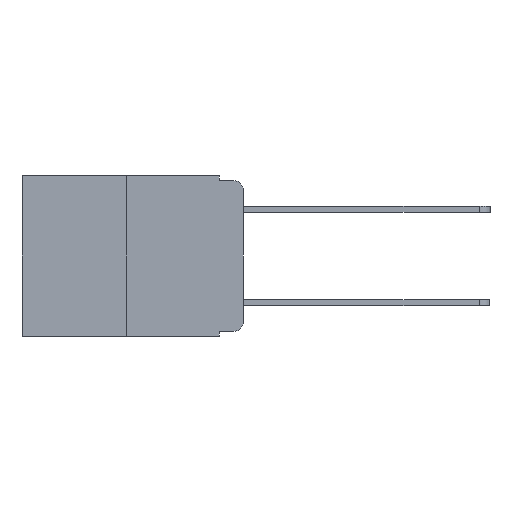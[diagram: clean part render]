
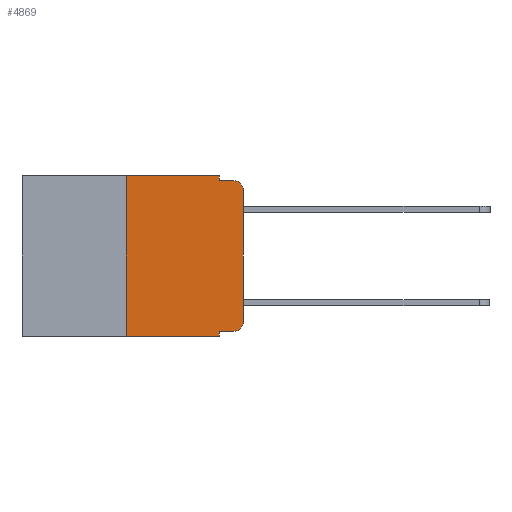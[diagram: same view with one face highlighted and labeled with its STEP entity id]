
A CAD part, left-side view. The second image highlights one B-rep face of the part: STEP entity #4869.
In plain terms, the highlighted planar face has unit normal (-1, 0, 0).
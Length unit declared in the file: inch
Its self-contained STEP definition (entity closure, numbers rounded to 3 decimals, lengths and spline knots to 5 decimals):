
#511 = LINE ( 'NONE', #5958, #3139 ) ;
#607 = ORIENTED_EDGE ( 'NONE', *, *, #5416, .T. ) ;
#632 = CARTESIAN_POINT ( 'NONE',  ( 0., 0.473, -0.343 ) ) ;
#1152 = VERTEX_POINT ( 'NONE', #1390 ) ;
#1154 = DIRECTION ( 'NONE',  ( 0., 0., -1. ) ) ;
#1282 = VERTEX_POINT ( 'NONE', #6256 ) ;
#1390 = CARTESIAN_POINT ( 'NONE',  ( 0., 0.02, -0.333 ) ) ;
#1535 = VECTOR ( 'NONE', #2801, 39.37008 ) ;
#1719 = EDGE_CURVE ( 'NONE', #7092, #6377, #4460, .T. ) ;
#1879 = VERTEX_POINT ( 'NONE', #2275 ) ;
#1970 = VECTOR ( 'NONE', #10909, 39.37008 ) ;
#1979 = CARTESIAN_POINT ( 'NONE',  ( 0., 0.02, -0.03 ) ) ;
#2105 = CARTESIAN_POINT ( 'NONE',  ( 0., 0.051, -0.343 ) ) ;
#2164 = CARTESIAN_POINT ( 'NONE',  ( 0., 0.051, -0.333 ) ) ;
#2275 = CARTESIAN_POINT ( 'NONE',  ( 0., 0.25, 0. ) ) ;
#2300 = AXIS2_PLACEMENT_3D ( 'NONE', #13156, #7542, #1154 ) ;
#2321 = CARTESIAN_POINT ( 'NONE',  ( 0., 0.051, -0.01 ) ) ;
#2801 = DIRECTION ( 'NONE',  ( 0., -1., 0. ) ) ;
#2997 = VERTEX_POINT ( 'NONE', #6821 ) ;
#3131 = VECTOR ( 'NONE', #5124, 39.37008 ) ;
#3139 = VECTOR ( 'NONE', #6002, 39.37008 ) ;
#3471 = CARTESIAN_POINT ( 'NONE',  ( 0., 0., -0.313 ) ) ;
#3485 = VERTEX_POINT ( 'NONE', #12842 ) ;
#3755 = PLANE ( 'NONE',  #7483 ) ;
#3914 = EDGE_CURVE ( 'NONE', #5323, #6377, #9899, .T. ) ;
#4236 = EDGE_LOOP ( 'NONE', ( #607, #6588, #8258, #5287, #4582, #8567, #7348, #9605, #12849, #6663 ) ) ;
#4460 = LINE ( 'NONE', #13046, #1535 ) ;
#4582 = ORIENTED_EDGE ( 'NONE', *, *, #7466, .F. ) ;
#4869 = ADVANCED_FACE ( 'NONE', ( #8647 ), #3755, .F. ) ;
#4973 = CARTESIAN_POINT ( 'NONE',  ( 0., 0., -0.03 ) ) ;
#5023 = VECTOR ( 'NONE', #10057, 39.37008 ) ;
#5072 = VECTOR ( 'NONE', #9431, 39.37008 ) ;
#5124 = DIRECTION ( 'NONE',  ( 0., 0., -1. ) ) ;
#5231 = LINE ( 'NONE', #9103, #1970 ) ;
#5278 = CIRCLE ( 'NONE', #2300, 0.02 ) ;
#5287 = ORIENTED_EDGE ( 'NONE', *, *, #12079, .F. ) ;
#5323 = VERTEX_POINT ( 'NONE', #4973 ) ;
#5416 = EDGE_CURVE ( 'NONE', #8509, #5323, #9421, .T. ) ;
#5656 = CARTESIAN_POINT ( 'NONE',  ( 0., 0., 0. ) ) ;
#5958 = CARTESIAN_POINT ( 'NONE',  ( 0., 0.25, 0. ) ) ;
#6002 = DIRECTION ( 'NONE',  ( 0., 0., 1. ) ) ;
#6009 = LINE ( 'NONE', #8120, #3131 ) ;
#6147 = CARTESIAN_POINT ( 'NONE',  ( 0., 0.473, 0. ) ) ;
#6256 = CARTESIAN_POINT ( 'NONE',  ( 0., 0.051, 0. ) ) ;
#6377 = VERTEX_POINT ( 'NONE', #7809 ) ;
#6547 = DIRECTION ( 'NONE',  ( 1., 0., 0. ) ) ;
#6588 = ORIENTED_EDGE ( 'NONE', *, *, #3914, .T. ) ;
#6663 = ORIENTED_EDGE ( 'NONE', *, *, #7675, .T. ) ;
#6821 = CARTESIAN_POINT ( 'NONE',  ( 0., 0.051, -0.333 ) ) ;
#7092 = VERTEX_POINT ( 'NONE', #2321 ) ;
#7214 = CARTESIAN_POINT ( 'NONE',  ( 0., 0.473, 0. ) ) ;
#7348 = ORIENTED_EDGE ( 'NONE', *, *, #10941, .T. ) ;
#7422 = VECTOR ( 'NONE', #12330, 39.37008 ) ;
#7466 = EDGE_CURVE ( 'NONE', #1879, #1282, #10366, .T. ) ;
#7483 = AXIS2_PLACEMENT_3D ( 'NONE', #6147, #6547, #7631 ) ;
#7542 = DIRECTION ( 'NONE',  ( -1., 0., 0. ) ) ;
#7631 = DIRECTION ( 'NONE',  ( 0., 0., -1. ) ) ;
#7675 = EDGE_CURVE ( 'NONE', #1152, #8509, #5278, .T. ) ;
#7781 = LINE ( 'NONE', #2164, #5072 ) ;
#7809 = CARTESIAN_POINT ( 'NONE',  ( 0., 0.02, -0.01 ) ) ;
#8120 = CARTESIAN_POINT ( 'NONE',  ( 0., 0.051, 0. ) ) ;
#8258 = ORIENTED_EDGE ( 'NONE', *, *, #1719, .F. ) ;
#8334 = EDGE_CURVE ( 'NONE', #2997, #1152, #7781, .T. ) ;
#8509 = VERTEX_POINT ( 'NONE', #3471 ) ;
#8517 = AXIS2_PLACEMENT_3D ( 'NONE', #1979, #10623, #10744 ) ;
#8567 = ORIENTED_EDGE ( 'NONE', *, *, #10856, .F. ) ;
#8647 = FACE_OUTER_BOUND ( 'NONE', #4236, .T. ) ;
#9103 = CARTESIAN_POINT ( 'NONE',  ( 0., 0.051, 0. ) ) ;
#9421 = LINE ( 'NONE', #5656, #7422 ) ;
#9431 = DIRECTION ( 'NONE',  ( 0., -1., 0. ) ) ;
#9605 = ORIENTED_EDGE ( 'NONE', *, *, #10277, .F. ) ;
#9724 = VERTEX_POINT ( 'NONE', #2105 ) ;
#9899 = CIRCLE ( 'NONE', #8517, 0.02 ) ;
#10057 = DIRECTION ( 'NONE',  ( 0., -1., 0. ) ) ;
#10135 = DIRECTION ( 'NONE',  ( 0., -1., 0. ) ) ;
#10277 = EDGE_CURVE ( 'NONE', #2997, #9724, #5231, .T. ) ;
#10366 = LINE ( 'NONE', #7214, #12770 ) ;
#10623 = DIRECTION ( 'NONE',  ( -1., 0., 0. ) ) ;
#10744 = DIRECTION ( 'NONE',  ( 0., 0., -1. ) ) ;
#10856 = EDGE_CURVE ( 'NONE', #3485, #1879, #511, .T. ) ;
#10909 = DIRECTION ( 'NONE',  ( 0., 0., -1. ) ) ;
#10941 = EDGE_CURVE ( 'NONE', #3485, #9724, #12703, .T. ) ;
#12079 = EDGE_CURVE ( 'NONE', #1282, #7092, #6009, .T. ) ;
#12330 = DIRECTION ( 'NONE',  ( 0., 0., 1. ) ) ;
#12703 = LINE ( 'NONE', #632, #5023 ) ;
#12770 = VECTOR ( 'NONE', #10135, 39.37008 ) ;
#12842 = CARTESIAN_POINT ( 'NONE',  ( 0., 0.25, -0.343 ) ) ;
#12849 = ORIENTED_EDGE ( 'NONE', *, *, #8334, .T. ) ;
#13046 = CARTESIAN_POINT ( 'NONE',  ( 0., 0.051, -0.01 ) ) ;
#13156 = CARTESIAN_POINT ( 'NONE',  ( 0., 0.02, -0.313 ) ) ;
